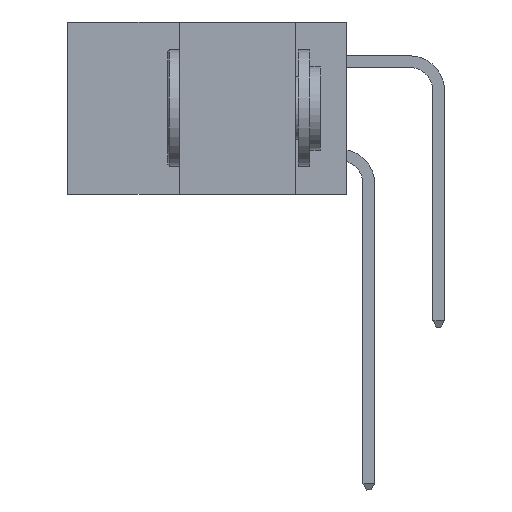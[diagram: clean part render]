
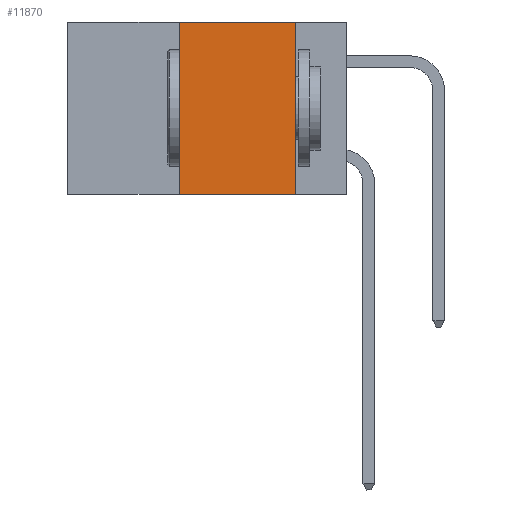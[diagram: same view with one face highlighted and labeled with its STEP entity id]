
A CAD part, left-side view. The second image highlights one B-rep face of the part: STEP entity #11870.
In plain terms, the highlighted planar face has unit normal (-1, 0, 0).
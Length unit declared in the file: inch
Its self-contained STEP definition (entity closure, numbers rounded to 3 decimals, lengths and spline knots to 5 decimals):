
#865 = EDGE_CURVE ( 'NONE', #7365, #5866, #14117, .T. ) ;
#1119 = VECTOR ( 'NONE', #21550, 39.37008 ) ;
#1259 = ORIENTED_EDGE ( 'NONE', *, *, #865, .F. ) ;
#1418 = DIRECTION ( 'NONE',  ( 0., 0., 1. ) ) ;
#1458 = LINE ( 'NONE', #21450, #10065 ) ;
#1586 = AXIS2_PLACEMENT_3D ( 'NONE', #1863, #3582, #15342 ) ;
#1863 = CARTESIAN_POINT ( 'NONE',  ( 0., 0.6, 0. ) ) ;
#1909 = CARTESIAN_POINT ( 'NONE',  ( 0., 0.6, 0. ) ) ;
#3065 = CARTESIAN_POINT ( 'NONE',  ( 0., 0.36, 0. ) ) ;
#3265 = DIRECTION ( 'NONE',  ( 0., -1., 0. ) ) ;
#3324 = VECTOR ( 'NONE', #3265, 39.37008 ) ;
#3464 = LINE ( 'NONE', #1909, #11995 ) ;
#3582 = DIRECTION ( 'NONE',  ( 1., 0., 0. ) ) ;
#3638 = DIRECTION ( 'NONE',  ( 0., -1., 0. ) ) ;
#3961 = ORIENTED_EDGE ( 'NONE', *, *, #9222, .F. ) ;
#5866 = VERTEX_POINT ( 'NONE', #21241 ) ;
#5976 = EDGE_LOOP ( 'NONE', ( #1259, #3961, #11182, #20679 ) ) ;
#6659 = EDGE_CURVE ( 'NONE', #11795, #5866, #16680, .T. ) ;
#7365 = VERTEX_POINT ( 'NONE', #12103 ) ;
#8253 = VERTEX_POINT ( 'NONE', #3065 ) ;
#9222 = EDGE_CURVE ( 'NONE', #8253, #7365, #3464, .T. ) ;
#10065 = VECTOR ( 'NONE', #1418, 39.37008 ) ;
#11182 = ORIENTED_EDGE ( 'NONE', *, *, #17483, .F. ) ;
#11795 = VERTEX_POINT ( 'NONE', #20075 ) ;
#11870 = ADVANCED_FACE ( 'NONE', ( #18194 ), #12070, .F. ) ;
#11995 = VECTOR ( 'NONE', #3638, 39.37008 ) ;
#12070 = PLANE ( 'NONE',  #1586 ) ;
#12103 = CARTESIAN_POINT ( 'NONE',  ( 0., 0.11, 0. ) ) ;
#14117 = LINE ( 'NONE', #21022, #1119 ) ;
#15342 = DIRECTION ( 'NONE',  ( 0., 0., -1. ) ) ;
#16680 = LINE ( 'NONE', #19913, #3324 ) ;
#17483 = EDGE_CURVE ( 'NONE', #11795, #8253, #1458, .T. ) ;
#18194 = FACE_OUTER_BOUND ( 'NONE', #5976, .T. ) ;
#19913 = CARTESIAN_POINT ( 'NONE',  ( 0., 0.6, -0.37 ) ) ;
#20075 = CARTESIAN_POINT ( 'NONE',  ( 0., 0.36, -0.37 ) ) ;
#20679 = ORIENTED_EDGE ( 'NONE', *, *, #6659, .T. ) ;
#21022 = CARTESIAN_POINT ( 'NONE',  ( 0., 0.11, 0. ) ) ;
#21241 = CARTESIAN_POINT ( 'NONE',  ( 0., 0.11, -0.37 ) ) ;
#21450 = CARTESIAN_POINT ( 'NONE',  ( 0., 0.36, 0. ) ) ;
#21550 = DIRECTION ( 'NONE',  ( 0., 0., -1. ) ) ;
